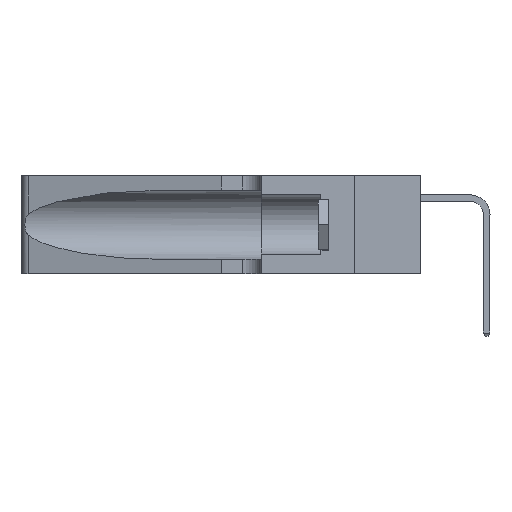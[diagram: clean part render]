
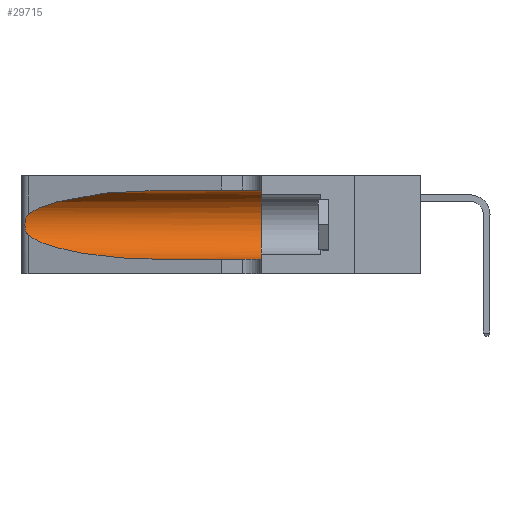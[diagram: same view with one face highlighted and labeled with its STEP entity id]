
A CAD part, left-side view. The second image highlights one B-rep face of the part: STEP entity #29715.
In plain terms, the highlighted cylindrical face has radius 3.308 mm (diameter 6.617 mm), a partial arc.
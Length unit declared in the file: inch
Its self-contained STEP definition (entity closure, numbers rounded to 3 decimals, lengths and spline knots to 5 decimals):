
#729 = CARTESIAN_POINT ( 'NONE',  ( 0.1305, 1.61858, 0.05475 ) ) ;
#1379 = CARTESIAN_POINT ( 'NONE',  ( 0.26075, 1.23896, 0.178 ) ) ;
#1415 = EDGE_CURVE ( 'NONE', #25907, #12389, #23950, .T. ) ;
#3350 = VERTEX_POINT ( 'NONE', #7031 ) ;
#4131 = CARTESIAN_POINT ( 'NONE',  ( 0.25555, 1.22994, 0.2215 ) ) ;
#4382 = CARTESIAN_POINT ( 'NONE',  ( 0.25856, 1.23593, 0.16098 ) ) ;
#5191 = CARTESIAN_POINT ( 'NONE',  ( 0.1305, 0.35, 0.185 ) ) ;
#7004 = EDGE_CURVE ( 'NONE', #12389, #9747, #21084, .T. ) ;
#7031 = CARTESIAN_POINT ( 'NONE',  ( 0.1305, 0.72297, 0.31525 ) ) ;
#7360 = CARTESIAN_POINT ( 'NONE',  ( 0.25639, 1.23186, 0.15144 ) ) ;
#7746 = DIRECTION ( 'NONE',  ( 0., 0., -1. ) ) ;
#7782 = CARTESIAN_POINT ( 'NONE',  ( 0.2373, 1.15595, 0.28018 ) ) ;
#8184 = DIRECTION ( 'NONE',  ( 0., 0., 1. ) ) ;
#9747 = VERTEX_POINT ( 'NONE', #30639 ) ;
#10140 = CARTESIAN_POINT ( 'NONE',  ( 0.2373, 1.15595, 0.08982 ) ) ;
#10422 = CARTESIAN_POINT ( 'NONE',  ( 0.25487, 1.22718, 0.14631 ) ) ;
#11735 = ORIENTED_EDGE ( 'NONE', *, *, #1415, .T. ) ;
#12389 = VERTEX_POINT ( 'NONE', #33537 ) ;
#13126 = CARTESIAN_POINT ( 'NONE',  ( 0.25487, 1.22718, 0.14631 ) ) ;
#13269 = CARTESIAN_POINT ( 'NONE',  ( 0.25639, 1.23184, 0.21858 ) ) ;
#14876 = CARTESIAN_POINT ( 'NONE',  ( 0.1305, 0.35, 0.31525 ) ) ;
#15366 = VERTEX_POINT ( 'NONE', #14876 ) ;
#15908 = EDGE_CURVE ( 'NONE', #15366, #34864, #24258, .T. ) ;
#16046 = CARTESIAN_POINT ( 'NONE',  ( 0.25487, 1.22718, 0.22369 ) ) ;
#16087 = CARTESIAN_POINT ( 'NONE',  ( 0.18966, 0.96281, 0.05475 ) ) ;
#16226 = CARTESIAN_POINT ( 'NONE',  ( 0.25854, 1.2359, 0.20912 ) ) ;
#16581 = EDGE_LOOP ( 'NONE', ( #30675, #11735, #37105, #24281, #32063, #22915 ) ) ;
#16653 = CARTESIAN_POINT ( 'NONE',  ( 0.1305, 0.72297, 0.31525 ) ) ;
#16751 = CARTESIAN_POINT ( 'NONE',  ( 0.1305, 1.61858, 0.185 ) ) ;
#17611 = VECTOR ( 'NONE', #18549, 39.37008 ) ;
#18549 = DIRECTION ( 'NONE',  ( 0., -1., 0. ) ) ;
#19233 = CARTESIAN_POINT ( 'NONE',  ( 0.26075, 1.23896, 0.19203 ) ) ;
#21084 =( BOUNDED_CURVE ( )  B_SPLINE_CURVE ( 3, ( #13126, #10140, #16087, #36698 ),
 .UNSPECIFIED., .F., .F. ) 
 B_SPLINE_CURVE_WITH_KNOTS ( ( 4, 4 ),
 ( 3.44316, 4.71239 ),
 .UNSPECIFIED. ) 
 CURVE ( )  GEOMETRIC_REPRESENTATION_ITEM ( )  RATIONAL_B_SPLINE_CURVE ( ( 1., 0.87, 0.87, 1. ) ) 
 REPRESENTATION_ITEM ( '' )  );
#22221 = CARTESIAN_POINT ( 'NONE',  ( 0.26017, 1.23833, 0.17102 ) ) ;
#22915 = ORIENTED_EDGE ( 'NONE', *, *, #33956, .F. ) ;
#23950 = B_SPLINE_CURVE_WITH_KNOTS ( 'NONE', 3,
 ( #28033, #4131, #13269, #33915, #16226, #36841, #19233, #1379, #22221, #4382, #25204, #7360, #28151, #10422 ),
 .UNSPECIFIED., .F., .F.,
 ( 4, 2, 2, 2, 2, 2, 4 ),
 ( 0., 0.00027, 0.00053, 0.00107, 0.0016, 0.00187, 0.00214 ),
 .UNSPECIFIED. ) ;
#24258 = CIRCLE ( 'NONE', #25036, 0.13025 ) ;
#24281 = ORIENTED_EDGE ( 'NONE', *, *, #35902, .T. ) ;
#24585 = DIRECTION ( 'NONE',  ( 0., -1., 0. ) ) ;
#25036 = AXIS2_PLACEMENT_3D ( 'NONE', #5191, #26013, #8184 ) ;
#25118 = AXIS2_PLACEMENT_3D ( 'NONE', #16751, #34408, #7746 ) ;
#25204 = CARTESIAN_POINT ( 'NONE',  ( 0.25789, 1.23486, 0.15765 ) ) ;
#25513 = LINE ( 'NONE', #33218, #17611 ) ;
#25907 = VERTEX_POINT ( 'NONE', #16046 ) ;
#26013 = DIRECTION ( 'NONE',  ( 0., 1., 0. ) ) ;
#28033 = CARTESIAN_POINT ( 'NONE',  ( 0.25487, 1.22718, 0.22369 ) ) ;
#28151 = CARTESIAN_POINT ( 'NONE',  ( 0.25555, 1.22993, 0.14849 ) ) ;
#28282 = VECTOR ( 'NONE', #24585, 39.37008 ) ;
#28546 = FACE_OUTER_BOUND ( 'NONE', #16581, .T. ) ;
#28562 = CARTESIAN_POINT ( 'NONE',  ( 0.25487, 1.22718, 0.22369 ) ) ;
#29715 = ADVANCED_FACE ( 'NONE', ( #28546 ), #35397, .F. ) ;
#30639 = CARTESIAN_POINT ( 'NONE',  ( 0.1305, 0.72297, 0.05475 ) ) ;
#30675 = ORIENTED_EDGE ( 'NONE', *, *, #31091, .T. ) ;
#31091 = EDGE_CURVE ( 'NONE', #3350, #25907, #35909, .T. ) ;
#31113 = CARTESIAN_POINT ( 'NONE',  ( 0.1305, 0.35, 0.05475 ) ) ;
#32063 = ORIENTED_EDGE ( 'NONE', *, *, #15908, .F. ) ;
#33218 = CARTESIAN_POINT ( 'NONE',  ( 0.1305, 1.61858, 0.31525 ) ) ;
#33537 = CARTESIAN_POINT ( 'NONE',  ( 0.25487, 1.22718, 0.14631 ) ) ;
#33915 = CARTESIAN_POINT ( 'NONE',  ( 0.25787, 1.23484, 0.2124 ) ) ;
#33956 = EDGE_CURVE ( 'NONE', #3350, #15366, #25513, .T. ) ;
#34322 = CARTESIAN_POINT ( 'NONE',  ( 0.18966, 0.96281, 0.31525 ) ) ;
#34408 = DIRECTION ( 'NONE',  ( 0., -1., 0. ) ) ;
#34864 = VERTEX_POINT ( 'NONE', #31113 ) ;
#35142 = LINE ( 'NONE', #729, #28282 ) ;
#35397 = CYLINDRICAL_SURFACE ( 'NONE', #25118, 0.13025 ) ;
#35902 = EDGE_CURVE ( 'NONE', #9747, #34864, #35142, .T. ) ;
#35909 =( BOUNDED_CURVE ( )  B_SPLINE_CURVE ( 3, ( #16653, #34322, #7782, #28562 ),
 .UNSPECIFIED., .F., .F. ) 
 B_SPLINE_CURVE_WITH_KNOTS ( ( 4, 4 ),
 ( 1.5708, 2.84003 ),
 .UNSPECIFIED. ) 
 CURVE ( )  GEOMETRIC_REPRESENTATION_ITEM ( )  RATIONAL_B_SPLINE_CURVE ( ( 1., 0.87, 0.87, 1. ) ) 
 REPRESENTATION_ITEM ( '' )  );
#36698 = CARTESIAN_POINT ( 'NONE',  ( 0.1305, 0.72297, 0.05475 ) ) ;
#36841 = CARTESIAN_POINT ( 'NONE',  ( 0.26018, 1.23835, 0.19895 ) ) ;
#37105 = ORIENTED_EDGE ( 'NONE', *, *, #7004, .T. ) ;
